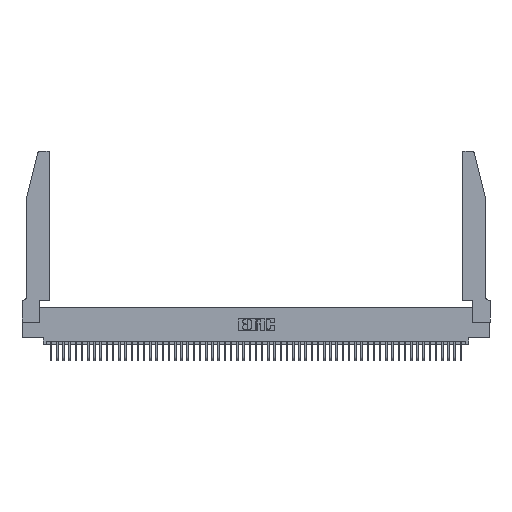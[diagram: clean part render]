
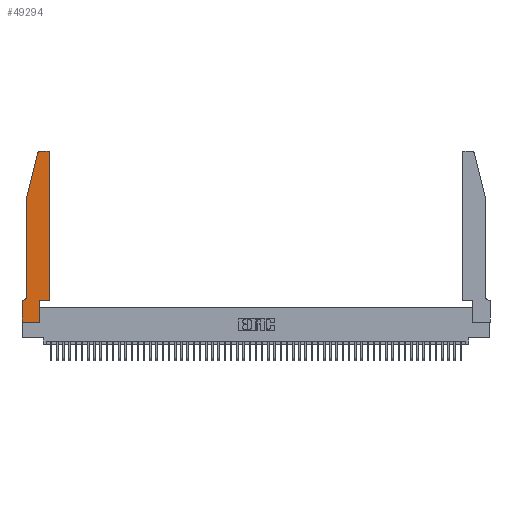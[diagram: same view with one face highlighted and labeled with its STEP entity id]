
A CAD part, top view. The second image highlights one B-rep face of the part: STEP entity #49294.
In plain terms, the highlighted planar face has unit normal (0, 0, 1).
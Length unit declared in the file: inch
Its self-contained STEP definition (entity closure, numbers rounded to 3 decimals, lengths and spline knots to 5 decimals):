
#831 = VERTEX_POINT ( 'NONE', #34720 ) ;
#963 = AXIS2_PLACEMENT_3D ( 'NONE', #41393, #17472, #45425 ) ;
#1980 = CARTESIAN_POINT ( 'NONE',  ( 0.0755, 2., 0.37 ) ) ;
#3222 = DIRECTION ( 'NONE',  ( -1., 0., 0. ) ) ;
#3547 = CARTESIAN_POINT ( 'NONE',  ( 0.4505, 0.35, 0.37 ) ) ;
#4099 = DIRECTION ( 'NONE',  ( 1., 0., 0. ) ) ;
#4157 = CARTESIAN_POINT ( 'NONE',  ( 0., 0., 0.37 ) ) ;
#4383 = ORIENTED_EDGE ( 'NONE', *, *, #44689, .T. ) ;
#4459 = DIRECTION ( 'NONE',  ( -1., 0., 0. ) ) ;
#5811 = EDGE_CURVE ( 'NONE', #50293, #22533, #32013, .T. ) ;
#6322 = CARTESIAN_POINT ( 'NONE',  ( 0., 0., 0.37 ) ) ;
#6845 = EDGE_CURVE ( 'NONE', #15432, #24014, #36245, .T. ) ;
#7571 = PLANE ( 'NONE',  #48084 ) ;
#7917 = VECTOR ( 'NONE', #28056, 39.37008 ) ;
#8266 = VECTOR ( 'NONE', #3222, 39.37008 ) ;
#9053 = VECTOR ( 'NONE', #51592, 39.37008 ) ;
#9140 = LINE ( 'NONE', #52008, #7917 ) ;
#9285 = CARTESIAN_POINT ( 'NONE',  ( 0.284, 2.75, 0.37 ) ) ;
#10480 = VERTEX_POINT ( 'NONE', #40929 ) ;
#10677 = ORIENTED_EDGE ( 'NONE', *, *, #45791, .T. ) ;
#10866 = EDGE_CURVE ( 'NONE', #24014, #10480, #40218, .T. ) ;
#11533 = CARTESIAN_POINT ( 'NONE',  ( 0.4505, 0.35, 0.37 ) ) ;
#11573 = VERTEX_POINT ( 'NONE', #48542 ) ;
#11603 = DIRECTION ( 'NONE',  ( 1., 0., 0. ) ) ;
#12330 = VERTEX_POINT ( 'NONE', #37093 ) ;
#12615 = CARTESIAN_POINT ( 'NONE',  ( 0.0055, 0.35, 0.37 ) ) ;
#13222 = CARTESIAN_POINT ( 'NONE',  ( 0.284, 2.72, 0.37 ) ) ;
#14304 = VECTOR ( 'NONE', #20706, 39.37008 ) ;
#14988 = FACE_OUTER_BOUND ( 'NONE', #45820, .T. ) ;
#15432 = VERTEX_POINT ( 'NONE', #18442 ) ;
#15938 = EDGE_CURVE ( 'NONE', #10480, #50293, #39029, .T. ) ;
#16353 = DIRECTION ( 'NONE',  ( 0., -1., 0. ) ) ;
#16600 = ORIENTED_EDGE ( 'NONE', *, *, #10866, .T. ) ;
#16624 = CARTESIAN_POINT ( 'NONE',  ( 0.4505, 0.35, 0.37 ) ) ;
#17260 = DIRECTION ( 'NONE',  ( 1., 0., 0. ) ) ;
#17355 = VERTEX_POINT ( 'NONE', #9285 ) ;
#17472 = DIRECTION ( 'NONE',  ( 0., 0., -1. ) ) ;
#17577 = CIRCLE ( 'NONE', #44316, 0.03 ) ;
#17589 = AXIS2_PLACEMENT_3D ( 'NONE', #20994, #48905, #25002 ) ;
#18442 = CARTESIAN_POINT ( 'NONE',  ( 0.0755, 0.42, 0.37 ) ) ;
#20706 = DIRECTION ( 'NONE',  ( 1., 0., 0. ) ) ;
#20960 = EDGE_CURVE ( 'NONE', #34851, #38264, #32929, .T. ) ;
#20994 = CARTESIAN_POINT ( 'NONE',  ( 0.4205, 2.72, 0.37 ) ) ;
#22533 = VERTEX_POINT ( 'NONE', #23498 ) ;
#23498 = CARTESIAN_POINT ( 'NONE',  ( 0.2865, 0., 0.37 ) ) ;
#24014 = VERTEX_POINT ( 'NONE', #12615 ) ;
#24440 = DIRECTION ( 'NONE',  ( -0.239, -0.971, 0. ) ) ;
#25002 = DIRECTION ( 'NONE',  ( 1., 0., 0. ) ) ;
#25186 = VECTOR ( 'NONE', #4459, 39.37008 ) ;
#25355 = VECTOR ( 'NONE', #34153, 39.37008 ) ;
#26400 = ORIENTED_EDGE ( 'NONE', *, *, #6845, .T. ) ;
#27210 = EDGE_CURVE ( 'NONE', #11573, #15432, #37179, .T. ) ;
#27314 = CARTESIAN_POINT ( 'NONE',  ( 0.0755, 0.35, 0.37 ) ) ;
#27607 = ORIENTED_EDGE ( 'NONE', *, *, #35486, .T. ) ;
#27921 = ORIENTED_EDGE ( 'NONE', *, *, #20960, .T. ) ;
#28056 = DIRECTION ( 'NONE',  ( 0., 1., 0. ) ) ;
#28419 = VECTOR ( 'NONE', #16353, 39.37008 ) ;
#28522 = CARTESIAN_POINT ( 'NONE',  ( 0.2605, 2.75, 0.37 ) ) ;
#28526 = ORIENTED_EDGE ( 'NONE', *, *, #29957, .T. ) ;
#28665 = EDGE_CURVE ( 'NONE', #28825, #11573, #30639, .T. ) ;
#28825 = VERTEX_POINT ( 'NONE', #49183 ) ;
#29377 = VECTOR ( 'NONE', #24440, 39.37008 ) ;
#29544 = CARTESIAN_POINT ( 'NONE',  ( 0.4505, 2.72, 0.37 ) ) ;
#29957 = EDGE_CURVE ( 'NONE', #22533, #831, #9140, .T. ) ;
#30639 = LINE ( 'NONE', #44339, #29377 ) ;
#30723 = VECTOR ( 'NONE', #4099, 39.37008 ) ;
#32013 = LINE ( 'NONE', #44268, #30723 ) ;
#32929 = LINE ( 'NONE', #3547, #9053 ) ;
#34104 = ORIENTED_EDGE ( 'NONE', *, *, #15938, .T. ) ;
#34153 = DIRECTION ( 'NONE',  ( 0., -1., 0. ) ) ;
#34720 = CARTESIAN_POINT ( 'NONE',  ( 0.2865, 0.35, 0.37 ) ) ;
#34851 = VERTEX_POINT ( 'NONE', #11533 ) ;
#35486 = EDGE_CURVE ( 'NONE', #38264, #12330, #41481, .T. ) ;
#35595 = DIRECTION ( 'NONE',  ( 0., 0., 1. ) ) ;
#36245 = CIRCLE ( 'NONE', #963, 0.07 ) ;
#36283 = EDGE_CURVE ( 'NONE', #12330, #17355, #45161, .T. ) ;
#36868 = ORIENTED_EDGE ( 'NONE', *, *, #5811, .T. ) ;
#37093 = CARTESIAN_POINT ( 'NONE',  ( 0.4205, 2.75, 0.37 ) ) ;
#37179 = LINE ( 'NONE', #1980, #25355 ) ;
#38264 = VERTEX_POINT ( 'NONE', #29544 ) ;
#39029 = LINE ( 'NONE', #4157, #28419 ) ;
#40218 = LINE ( 'NONE', #27314, #8266 ) ;
#40929 = CARTESIAN_POINT ( 'NONE',  ( 0., 0.35, 0.37 ) ) ;
#41185 = DIRECTION ( 'NONE',  ( 0., 0., 1. ) ) ;
#41393 = CARTESIAN_POINT ( 'NONE',  ( 0.0055, 0.42, 0.37 ) ) ;
#41481 = CIRCLE ( 'NONE', #17589, 0.03 ) ;
#42700 = ORIENTED_EDGE ( 'NONE', *, *, #27210, .T. ) ;
#43477 = CARTESIAN_POINT ( 'NONE',  ( 0., 0.35, 0.37 ) ) ;
#44268 = CARTESIAN_POINT ( 'NONE',  ( 0., 0., 0.37 ) ) ;
#44316 = AXIS2_PLACEMENT_3D ( 'NONE', #13222, #41185, #17260 ) ;
#44339 = CARTESIAN_POINT ( 'NONE',  ( 0.0755, 2., 0.37 ) ) ;
#44689 = EDGE_CURVE ( 'NONE', #17355, #28825, #17577, .T. ) ;
#45161 = LINE ( 'NONE', #28522, #25186 ) ;
#45425 = DIRECTION ( 'NONE',  ( -1., 0., 0. ) ) ;
#45791 = EDGE_CURVE ( 'NONE', #831, #34851, #46195, .T. ) ;
#45820 = EDGE_LOOP ( 'NONE', ( #49783, #4383, #47208, #42700, #26400, #16600, #34104, #36868, #28526, #10677, #27921, #27607 ) ) ;
#46195 = LINE ( 'NONE', #16624, #14304 ) ;
#47208 = ORIENTED_EDGE ( 'NONE', *, *, #28665, .T. ) ;
#48084 = AXIS2_PLACEMENT_3D ( 'NONE', #43477, #35595, #11603 ) ;
#48542 = CARTESIAN_POINT ( 'NONE',  ( 0.0755, 2., 0.37 ) ) ;
#48905 = DIRECTION ( 'NONE',  ( 0., 0., 1. ) ) ;
#49183 = CARTESIAN_POINT ( 'NONE',  ( 0.25487, 2.72718, 0.37 ) ) ;
#49294 = ADVANCED_FACE ( 'NONE', ( #14988 ), #7571, .T. ) ;
#49783 = ORIENTED_EDGE ( 'NONE', *, *, #36283, .T. ) ;
#50293 = VERTEX_POINT ( 'NONE', #6322 ) ;
#51592 = DIRECTION ( 'NONE',  ( 0., 1., 0. ) ) ;
#52008 = CARTESIAN_POINT ( 'NONE',  ( 0.2865, 0.35, 0.37 ) ) ;
